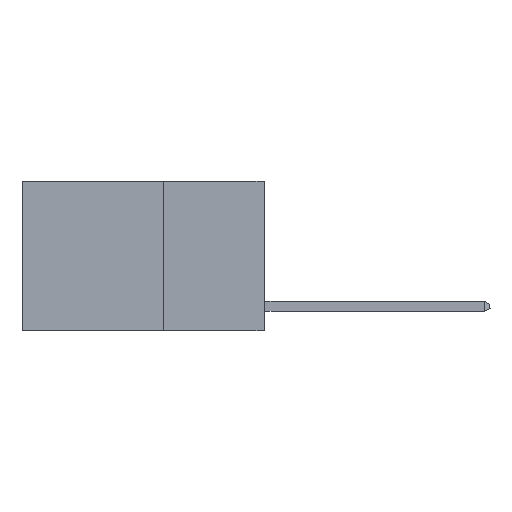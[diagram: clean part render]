
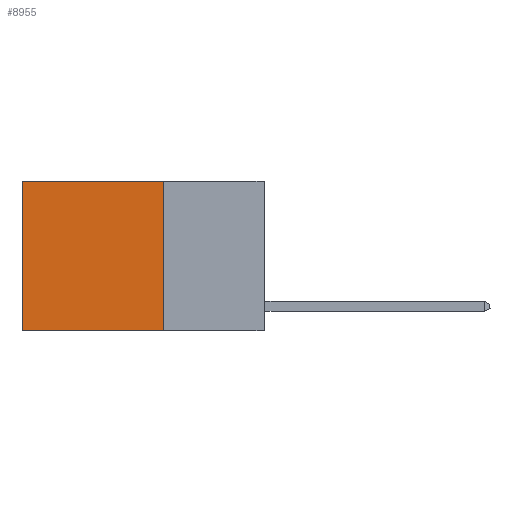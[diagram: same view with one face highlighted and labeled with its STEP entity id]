
A CAD part, left-side view. The second image highlights one B-rep face of the part: STEP entity #8955.
In plain terms, the highlighted planar face has unit normal (-1, 0, 0).
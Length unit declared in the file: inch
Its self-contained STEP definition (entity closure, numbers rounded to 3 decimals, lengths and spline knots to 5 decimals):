
#637 = VECTOR ( 'NONE', #6582, 39.37008 ) ;
#1100 = EDGE_CURVE ( 'NONE', #6947, #8298, #11470, .T. ) ;
#1253 = CARTESIAN_POINT ( 'NONE',  ( 0.2625, 0.6, 0. ) ) ;
#1865 = CARTESIAN_POINT ( 'NONE',  ( 0.2625, 0.25, 0. ) ) ;
#2622 = EDGE_CURVE ( 'NONE', #6947, #13661, #15742, .T. ) ;
#3279 = DIRECTION ( 'NONE',  ( 0., 0., -1. ) ) ;
#3444 = DIRECTION ( 'NONE',  ( 1., 0., 0. ) ) ;
#3459 = ORIENTED_EDGE ( 'NONE', *, *, #4067, .F. ) ;
#4067 = EDGE_CURVE ( 'NONE', #8298, #8184, #7863, .T. ) ;
#4298 = VECTOR ( 'NONE', #3279, 39.37008 ) ;
#4832 = CARTESIAN_POINT ( 'NONE',  ( 0.2625, 0.25, 0. ) ) ;
#5055 = CARTESIAN_POINT ( 'NONE',  ( 0.2625, 0.25, -0.37 ) ) ;
#5178 = FACE_OUTER_BOUND ( 'NONE', #6683, .T. ) ;
#6582 = DIRECTION ( 'NONE',  ( 0., 1., 0. ) ) ;
#6683 = EDGE_LOOP ( 'NONE', ( #10564, #3459, #13200, #15699 ) ) ;
#6828 = CARTESIAN_POINT ( 'NONE',  ( 0.2625, 0.6, 0. ) ) ;
#6869 = LINE ( 'NONE', #1253, #7282 ) ;
#6947 = VERTEX_POINT ( 'NONE', #1865 ) ;
#7282 = VECTOR ( 'NONE', #10707, 39.37008 ) ;
#7493 = CARTESIAN_POINT ( 'NONE',  ( 0.2625, 0.25, 0. ) ) ;
#7863 = LINE ( 'NONE', #5055, #637 ) ;
#8184 = VERTEX_POINT ( 'NONE', #15117 ) ;
#8298 = VERTEX_POINT ( 'NONE', #11559 ) ;
#8851 = PLANE ( 'NONE',  #15962 ) ;
#8955 = ADVANCED_FACE ( 'NONE', ( #5178 ), #8851, .F. ) ;
#10564 = ORIENTED_EDGE ( 'NONE', *, *, #11410, .T. ) ;
#10707 = DIRECTION ( 'NONE',  ( 0., 0., -1. ) ) ;
#11410 = EDGE_CURVE ( 'NONE', #13661, #8184, #6869, .T. ) ;
#11470 = LINE ( 'NONE', #4832, #4298 ) ;
#11559 = CARTESIAN_POINT ( 'NONE',  ( 0.2625, 0.25, -0.37 ) ) ;
#12220 = VECTOR ( 'NONE', #14937, 39.37008 ) ;
#12858 = DIRECTION ( 'NONE',  ( 0., 0., -1. ) ) ;
#12969 = CARTESIAN_POINT ( 'NONE',  ( 0.2625, 0.25, 0. ) ) ;
#13200 = ORIENTED_EDGE ( 'NONE', *, *, #1100, .F. ) ;
#13661 = VERTEX_POINT ( 'NONE', #6828 ) ;
#14937 = DIRECTION ( 'NONE',  ( 0., 1., 0. ) ) ;
#15117 = CARTESIAN_POINT ( 'NONE',  ( 0.2625, 0.6, -0.37 ) ) ;
#15699 = ORIENTED_EDGE ( 'NONE', *, *, #2622, .T. ) ;
#15742 = LINE ( 'NONE', #12969, #12220 ) ;
#15962 = AXIS2_PLACEMENT_3D ( 'NONE', #7493, #3444, #12858 ) ;
